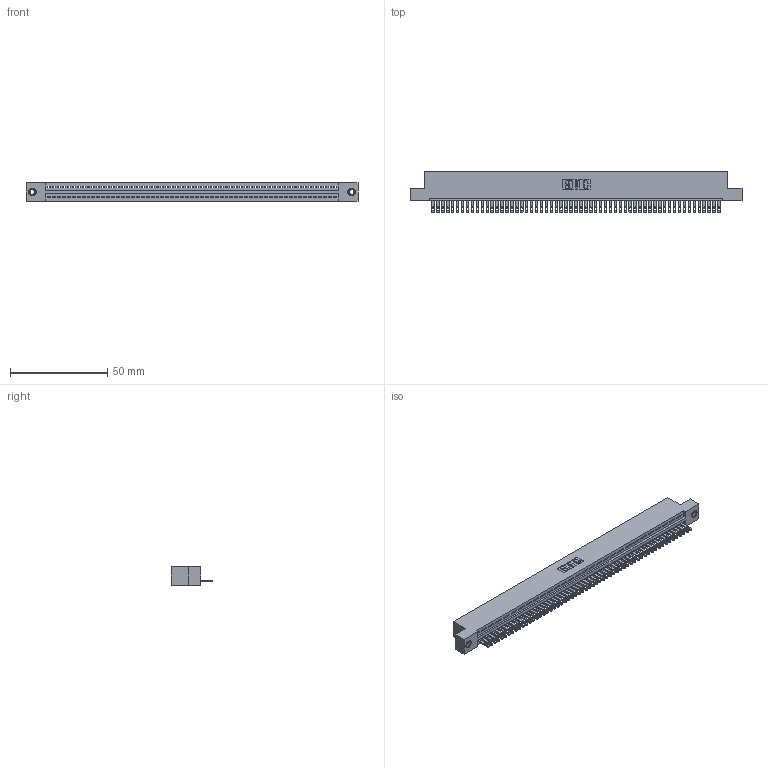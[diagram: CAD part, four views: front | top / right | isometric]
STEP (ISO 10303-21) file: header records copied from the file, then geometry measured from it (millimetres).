
FILE_DESCRIPTION (( 'STEP AP203' ), '1' );
FILE_NAME ('895-059-500-107.STEP', '2020-09-28T03:45:41', ( '' ), ( '' ), 'SwSTEP 2.0', 'SolidWorks 2020', '' );
FILE_SCHEMA (( 'CONFIG_CONTROL_DESIGN' ));
Length unit declared in the file: inch
Products named in the file (4): 845 Part_Flush Mounting Lugs - 0.156 Dia-TI; 345-292-001_345-293-100; 345-250-001_345-250-005-103; 895-059-500-107
Assembly tree (62 placements, depth 2):
  895-059-500-107
    845 Part_Flush Mounting Lugs - 0.156 Dia-TI
    345-292-001_345-293-100  x59
    345-250-001_345-250-005-103  x2
Bounding box: 171.07 x 21.51 x 9.4 mm (x, y, z)
Volume: 16410.6 mm3; surface area: 22204.3 mm2
Topology: 62 solids, 62 shells, 3372 faces, 10389 edges, 6918 vertices
Faces by surface type: plane 2118, cylinder 1238, cone 12, torus 4
Entity records: 43232 total; most frequent: CARTESIAN_POINT 7468, ORIENTED_EDGE 7454, DIRECTION 6527, EDGE_CURVE 3727, LINE 3335, VECTOR 3335, VERTEX_POINT 2480, AXIS2_PLACEMENT_3D 1596
